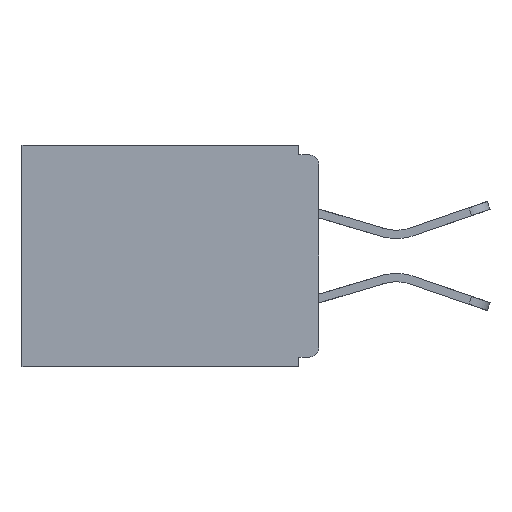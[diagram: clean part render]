
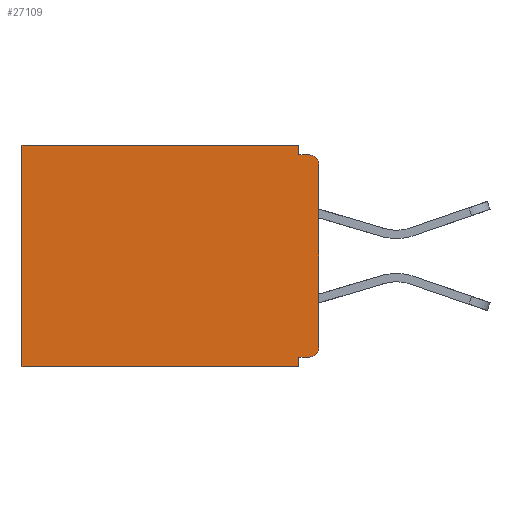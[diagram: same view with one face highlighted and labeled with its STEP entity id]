
A CAD part, left-side view. The second image highlights one B-rep face of the part: STEP entity #27109.
In plain terms, the highlighted planar face has unit normal (-1, 0, 0).
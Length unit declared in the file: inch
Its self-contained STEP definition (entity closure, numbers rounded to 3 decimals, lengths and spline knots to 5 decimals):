
#46 = ORIENTED_EDGE ( 'NONE', *, *, #23840, .T. ) ;
#48 = LINE ( 'NONE', #15610, #20670 ) ;
#502 = CIRCLE ( 'NONE', #22895, 0.015 ) ;
#519 = VERTEX_POINT ( 'NONE', #12305 ) ;
#572 = CARTESIAN_POINT ( 'NONE',  ( 0.298, 0., 0. ) ) ;
#889 = DIRECTION ( 'NONE',  ( 0., 0., -1. ) ) ;
#1049 = ORIENTED_EDGE ( 'NONE', *, *, #5274, .T. ) ;
#1983 = EDGE_CURVE ( 'NONE', #22681, #21615, #25873, .T. ) ;
#2060 = DIRECTION ( 'NONE',  ( 0., -1., 0. ) ) ;
#2274 = LINE ( 'NONE', #25010, #28251 ) ;
#2676 = LINE ( 'NONE', #11463, #6247 ) ;
#2861 = DIRECTION ( 'NONE',  ( 1., 0., 0. ) ) ;
#2902 = EDGE_CURVE ( 'NONE', #21615, #10240, #9001, .T. ) ;
#3210 = DIRECTION ( 'NONE',  ( 0., 0., -1. ) ) ;
#3343 = LINE ( 'NONE', #572, #14413 ) ;
#3951 = CARTESIAN_POINT ( 'NONE',  ( 0.298, 0.031, -0.015 ) ) ;
#4295 = LINE ( 'NONE', #23733, #23468 ) ;
#4950 = DIRECTION ( 'NONE',  ( -1., 0., 0. ) ) ;
#5040 = DIRECTION ( 'NONE',  ( 0., 0., -1. ) ) ;
#5274 = EDGE_CURVE ( 'NONE', #28763, #8881, #4295, .T. ) ;
#5344 = EDGE_CURVE ( 'NONE', #17865, #13577, #12867, .T. ) ;
#6201 = AXIS2_PLACEMENT_3D ( 'NONE', #20076, #8506, #24627 ) ;
#6247 = VECTOR ( 'NONE', #18552, 39.37008 ) ;
#6305 = VECTOR ( 'NONE', #20129, 39.37008 ) ;
#7921 = ORIENTED_EDGE ( 'NONE', *, *, #2902, .F. ) ;
#7955 = ORIENTED_EDGE ( 'NONE', *, *, #1983, .F. ) ;
#8423 = VECTOR ( 'NONE', #3210, 39.37008 ) ;
#8506 = DIRECTION ( 'NONE',  ( -1., 0., 0. ) ) ;
#8849 = EDGE_CURVE ( 'NONE', #17865, #22681, #2676, .T. ) ;
#8881 = VERTEX_POINT ( 'NONE', #13941 ) ;
#9001 = LINE ( 'NONE', #20576, #23277 ) ;
#9223 = VERTEX_POINT ( 'NONE', #3951 ) ;
#9230 = ORIENTED_EDGE ( 'NONE', *, *, #11794, .F. ) ;
#9545 = FACE_OUTER_BOUND ( 'NONE', #16820, .T. ) ;
#10240 = VERTEX_POINT ( 'NONE', #26084 ) ;
#11463 = CARTESIAN_POINT ( 'NONE',  ( 0.298, 0., -0.328 ) ) ;
#11649 = CARTESIAN_POINT ( 'NONE',  ( 0.298, 0.031, -0.328 ) ) ;
#11794 = EDGE_CURVE ( 'NONE', #9223, #519, #48, .T. ) ;
#12305 = CARTESIAN_POINT ( 'NONE',  ( 0.298, 0.015, -0.015 ) ) ;
#12820 = CARTESIAN_POINT ( 'NONE',  ( 0.298, 0.031, 0. ) ) ;
#12867 = CIRCLE ( 'NONE', #6201, 0.015 ) ;
#13577 = VERTEX_POINT ( 'NONE', #27129 ) ;
#13643 = DIRECTION ( 'NONE',  ( 0., 0., -1. ) ) ;
#13941 = CARTESIAN_POINT ( 'NONE',  ( 0.298, 0.46, 0. ) ) ;
#14413 = VECTOR ( 'NONE', #5040, 39.37008 ) ;
#14563 = CARTESIAN_POINT ( 'NONE',  ( 0.298, 0.031, -0.343 ) ) ;
#15610 = CARTESIAN_POINT ( 'NONE',  ( 0.298, 0., -0.015 ) ) ;
#16261 = DIRECTION ( 'NONE',  ( 0., 1., 0. ) ) ;
#16702 = DIRECTION ( 'NONE',  ( 0., 0., -1. ) ) ;
#16820 = EDGE_LOOP ( 'NONE', ( #28727, #9230, #17946, #1049, #46, #7921, #7955, #19140, #25370, #23722 ) ) ;
#17546 = VERTEX_POINT ( 'NONE', #22389 ) ;
#17784 = EDGE_CURVE ( 'NONE', #17546, #519, #502, .T. ) ;
#17865 = VERTEX_POINT ( 'NONE', #22450 ) ;
#17946 = ORIENTED_EDGE ( 'NONE', *, *, #28035, .F. ) ;
#18552 = DIRECTION ( 'NONE',  ( 0., 1., 0. ) ) ;
#18774 = CARTESIAN_POINT ( 'NONE',  ( 0.298, 0.015, -0.03 ) ) ;
#18779 = DIRECTION ( 'NONE',  ( 0., 1., 0. ) ) ;
#19140 = ORIENTED_EDGE ( 'NONE', *, *, #8849, .F. ) ;
#20076 = CARTESIAN_POINT ( 'NONE',  ( 0.298, 0.015, -0.313 ) ) ;
#20129 = DIRECTION ( 'NONE',  ( 0., 0., -1. ) ) ;
#20424 = CARTESIAN_POINT ( 'NONE',  ( 0.298, 0.031, -0.343 ) ) ;
#20576 = CARTESIAN_POINT ( 'NONE',  ( 0.298, 0., -0.343 ) ) ;
#20670 = VECTOR ( 'NONE', #2060, 39.37008 ) ;
#21615 = VERTEX_POINT ( 'NONE', #21744 ) ;
#21744 = CARTESIAN_POINT ( 'NONE',  ( 0.298, 0.031, -0.343 ) ) ;
#22389 = CARTESIAN_POINT ( 'NONE',  ( 0.298, 0., -0.03 ) ) ;
#22450 = CARTESIAN_POINT ( 'NONE',  ( 0.298, 0.015, -0.328 ) ) ;
#22681 = VERTEX_POINT ( 'NONE', #11649 ) ;
#22895 = AXIS2_PLACEMENT_3D ( 'NONE', #18774, #4950, #16702 ) ;
#23277 = VECTOR ( 'NONE', #16261, 39.37008 ) ;
#23468 = VECTOR ( 'NONE', #18779, 39.37008 ) ;
#23470 = AXIS2_PLACEMENT_3D ( 'NONE', #27918, #2861, #889 ) ;
#23550 = PLANE ( 'NONE',  #23470 ) ;
#23719 = LINE ( 'NONE', #14563, #8423 ) ;
#23722 = ORIENTED_EDGE ( 'NONE', *, *, #23800, .F. ) ;
#23733 = CARTESIAN_POINT ( 'NONE',  ( 0.298, 0., 0. ) ) ;
#23800 = EDGE_CURVE ( 'NONE', #17546, #13577, #3343, .T. ) ;
#23840 = EDGE_CURVE ( 'NONE', #8881, #10240, #2274, .T. ) ;
#24627 = DIRECTION ( 'NONE',  ( 0., 0., -1. ) ) ;
#25010 = CARTESIAN_POINT ( 'NONE',  ( 0.298, 0.46, 0. ) ) ;
#25370 = ORIENTED_EDGE ( 'NONE', *, *, #5344, .T. ) ;
#25873 = LINE ( 'NONE', #20424, #6305 ) ;
#26084 = CARTESIAN_POINT ( 'NONE',  ( 0.298, 0.46, -0.343 ) ) ;
#27109 = ADVANCED_FACE ( 'NONE', ( #9545 ), #23550, .F. ) ;
#27129 = CARTESIAN_POINT ( 'NONE',  ( 0.298, 0., -0.313 ) ) ;
#27918 = CARTESIAN_POINT ( 'NONE',  ( 0.298, 0., 0. ) ) ;
#28035 = EDGE_CURVE ( 'NONE', #28763, #9223, #23719, .T. ) ;
#28251 = VECTOR ( 'NONE', #13643, 39.37008 ) ;
#28727 = ORIENTED_EDGE ( 'NONE', *, *, #17784, .T. ) ;
#28763 = VERTEX_POINT ( 'NONE', #12820 ) ;
